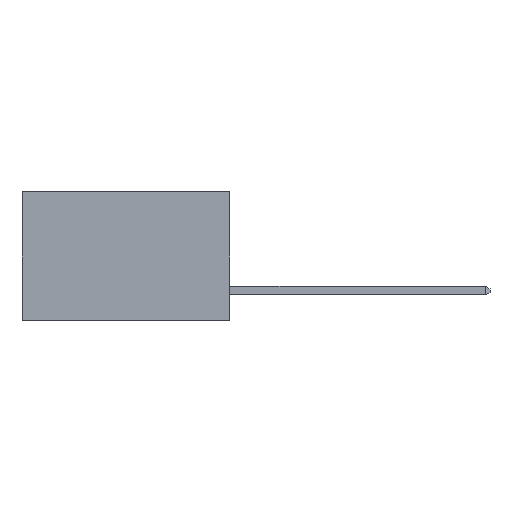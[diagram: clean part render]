
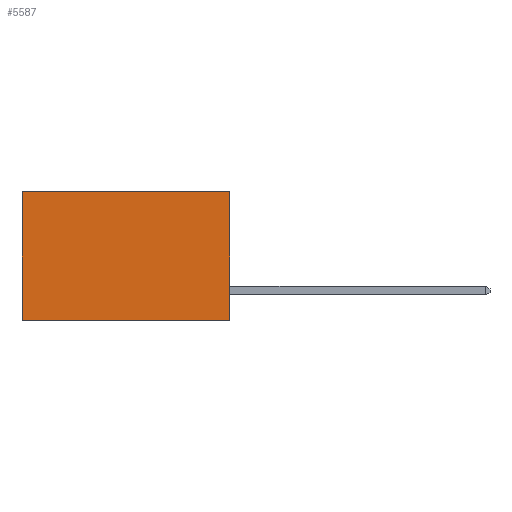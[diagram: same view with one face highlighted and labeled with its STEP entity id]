
A CAD part, left-side view. The second image highlights one B-rep face of the part: STEP entity #5587.
In plain terms, the highlighted planar face has unit normal (-1, 0, 0).
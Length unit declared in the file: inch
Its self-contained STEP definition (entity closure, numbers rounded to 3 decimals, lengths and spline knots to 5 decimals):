
#120 = FACE_OUTER_BOUND ( 'NONE', #6591, .T. ) ;
#814 = VECTOR ( 'NONE', #6171, 39.37008 ) ;
#1396 = AXIS2_PLACEMENT_3D ( 'NONE', #10679, #10669, #9289 ) ;
#2065 = CARTESIAN_POINT ( 'NONE',  ( 0.2615, 0., 0. ) ) ;
#2127 = EDGE_CURVE ( 'NONE', #4362, #4261, #6169, .T. ) ;
#2152 = EDGE_CURVE ( 'NONE', #2698, #4261, #5907, .T. ) ;
#2636 = CARTESIAN_POINT ( 'NONE',  ( 0.2615, 0.6, 0. ) ) ;
#2698 = VERTEX_POINT ( 'NONE', #2636 ) ;
#3363 = ORIENTED_EDGE ( 'NONE', *, *, #2152, .T. ) ;
#3397 = ORIENTED_EDGE ( 'NONE', *, *, #2127, .F. ) ;
#3419 = ORIENTED_EDGE ( 'NONE', *, *, #5147, .F. ) ;
#3459 = ORIENTED_EDGE ( 'NONE', *, *, #9916, .T. ) ;
#4015 = CARTESIAN_POINT ( 'NONE',  ( 0.2615, 0.6, -0.37 ) ) ;
#4261 = VERTEX_POINT ( 'NONE', #4015 ) ;
#4362 = VERTEX_POINT ( 'NONE', #8386 ) ;
#5147 = EDGE_CURVE ( 'NONE', #8364, #4362, #9010, .T. ) ;
#5587 = ADVANCED_FACE ( 'NONE', ( #120 ), #10691, .F. ) ;
#5907 = LINE ( 'NONE', #10517, #10085 ) ;
#6169 = LINE ( 'NONE', #10660, #8169 ) ;
#6171 = DIRECTION ( 'NONE',  ( 0., 1., 0. ) ) ;
#6591 = EDGE_LOOP ( 'NONE', ( #3363, #3397, #3419, #3459 ) ) ;
#8002 = CARTESIAN_POINT ( 'NONE',  ( 0.2615, 0., -0.37 ) ) ;
#8038 = DIRECTION ( 'NONE',  ( 0., 0., -1. ) ) ;
#8169 = VECTOR ( 'NONE', #10572, 39.37008 ) ;
#8364 = VERTEX_POINT ( 'NONE', #2065 ) ;
#8386 = CARTESIAN_POINT ( 'NONE',  ( 0.2615, 0., -0.37 ) ) ;
#8752 = VECTOR ( 'NONE', #8038, 39.37008 ) ;
#9010 = LINE ( 'NONE', #8002, #8752 ) ;
#9289 = DIRECTION ( 'NONE',  ( 0., 0., -1. ) ) ;
#9804 = LINE ( 'NONE', #10315, #814 ) ;
#9916 = EDGE_CURVE ( 'NONE', #8364, #2698, #9804, .T. ) ;
#10085 = VECTOR ( 'NONE', #10232, 39.37008 ) ;
#10232 = DIRECTION ( 'NONE',  ( 0., 0., -1. ) ) ;
#10315 = CARTESIAN_POINT ( 'NONE',  ( 0.2615, 0., 0. ) ) ;
#10517 = CARTESIAN_POINT ( 'NONE',  ( 0.2615, 0.6, -0.37 ) ) ;
#10572 = DIRECTION ( 'NONE',  ( 0., 1., 0. ) ) ;
#10660 = CARTESIAN_POINT ( 'NONE',  ( 0.2615, 0., -0.37 ) ) ;
#10669 = DIRECTION ( 'NONE',  ( 1., 0., 0. ) ) ;
#10679 = CARTESIAN_POINT ( 'NONE',  ( 0.2615, 0., -0.37 ) ) ;
#10691 = PLANE ( 'NONE',  #1396 ) ;
